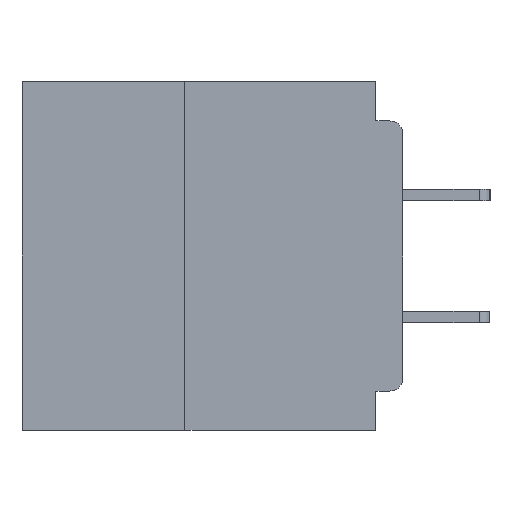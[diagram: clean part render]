
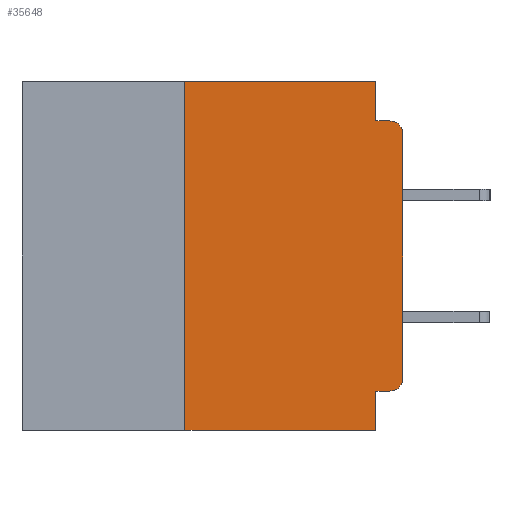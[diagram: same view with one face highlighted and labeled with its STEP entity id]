
A CAD part, left-side view. The second image highlights one B-rep face of the part: STEP entity #35648.
In plain terms, the highlighted planar face has unit normal (-1, 0, 0).
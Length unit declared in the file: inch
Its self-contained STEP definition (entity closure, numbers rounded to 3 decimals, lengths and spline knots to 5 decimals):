
#379 = EDGE_CURVE ( 'NONE', #28760, #12139, #10745, .T. ) ;
#477 = DIRECTION ( 'NONE',  ( 0., 0., 1. ) ) ;
#752 = VECTOR ( 'NONE', #17042, 39.37008 ) ;
#1102 = EDGE_CURVE ( 'NONE', #30086, #15350, #31652, .T. ) ;
#1148 = CARTESIAN_POINT ( 'NONE',  ( 0., 0.25, -0.4 ) ) ;
#1332 = ORIENTED_EDGE ( 'NONE', *, *, #379, .F. ) ;
#1874 = VECTOR ( 'NONE', #34496, 39.37008 ) ;
#2304 = DIRECTION ( 'NONE',  ( 0., 1., 0. ) ) ;
#2606 = LINE ( 'NONE', #16380, #752 ) ;
#2847 = CARTESIAN_POINT ( 'NONE',  ( 0., 0., -0.355 ) ) ;
#2951 = DIRECTION ( 'NONE',  ( 0., -1., 0. ) ) ;
#3468 = DIRECTION ( 'NONE',  ( 1., 0., 0. ) ) ;
#3706 = CARTESIAN_POINT ( 'NONE',  ( 0., 0.031, -0.4 ) ) ;
#4306 = VECTOR ( 'NONE', #2951, 39.37008 ) ;
#4552 = ORIENTED_EDGE ( 'NONE', *, *, #7566, .F. ) ;
#5007 = CARTESIAN_POINT ( 'NONE',  ( 0., 0., -0.34 ) ) ;
#5410 = EDGE_CURVE ( 'NONE', #15923, #11881, #2606, .T. ) ;
#6106 = ORIENTED_EDGE ( 'NONE', *, *, #32459, .T. ) ;
#6788 = EDGE_CURVE ( 'NONE', #8379, #30281, #9928, .T. ) ;
#7203 = EDGE_CURVE ( 'NONE', #11881, #18662, #31814, .T. ) ;
#7566 = EDGE_CURVE ( 'NONE', #12412, #28760, #35286, .T. ) ;
#7842 = EDGE_CURVE ( 'NONE', #30281, #18662, #17129, .T. ) ;
#7962 = EDGE_CURVE ( 'NONE', #12412, #8379, #21242, .T. ) ;
#7987 = CARTESIAN_POINT ( 'NONE',  ( 0., 0.015, -0.045 ) ) ;
#8293 = ORIENTED_EDGE ( 'NONE', *, *, #1102, .F. ) ;
#8379 = VERTEX_POINT ( 'NONE', #5007 ) ;
#8835 = DIRECTION ( 'NONE',  ( 0., 0., -1. ) ) ;
#8938 = CARTESIAN_POINT ( 'NONE',  ( 0., 0.031, -0.045 ) ) ;
#8981 = DIRECTION ( 'NONE',  ( -1., 0., 0. ) ) ;
#9009 = CARTESIAN_POINT ( 'NONE',  ( 0., 0.015, -0.34 ) ) ;
#9731 = VECTOR ( 'NONE', #477, 39.37008 ) ;
#9914 = DIRECTION ( 'NONE',  ( 0., 0., 1. ) ) ;
#9928 = LINE ( 'NONE', #10105, #16770 ) ;
#10105 = CARTESIAN_POINT ( 'NONE',  ( 0., 0., 0. ) ) ;
#10274 = AXIS2_PLACEMENT_3D ( 'NONE', #17454, #17327, #17278 ) ;
#10745 = LINE ( 'NONE', #3706, #1874 ) ;
#10954 = ORIENTED_EDGE ( 'NONE', *, *, #5410, .F. ) ;
#11767 = CARTESIAN_POINT ( 'NONE',  ( 0., 0., -0.06 ) ) ;
#11881 = VERTEX_POINT ( 'NONE', #8938 ) ;
#12139 = VERTEX_POINT ( 'NONE', #36090 ) ;
#12412 = VERTEX_POINT ( 'NONE', #23268 ) ;
#12606 = VECTOR ( 'NONE', #2304, 39.37008 ) ;
#13993 = ORIENTED_EDGE ( 'NONE', *, *, #29779, .F. ) ;
#14252 = ORIENTED_EDGE ( 'NONE', *, *, #6788, .T. ) ;
#15350 = VERTEX_POINT ( 'NONE', #33394 ) ;
#15496 = ORIENTED_EDGE ( 'NONE', *, *, #7203, .F. ) ;
#15923 = VERTEX_POINT ( 'NONE', #21851 ) ;
#15999 = CARTESIAN_POINT ( 'NONE',  ( 0., 0., -0.045 ) ) ;
#16330 = DIRECTION ( 'NONE',  ( 0., -1., 0. ) ) ;
#16375 = DIRECTION ( 'NONE',  ( 0., -1., 0. ) ) ;
#16380 = CARTESIAN_POINT ( 'NONE',  ( 0., 0.031, 0. ) ) ;
#16607 = VECTOR ( 'NONE', #16330, 39.37008 ) ;
#16770 = VECTOR ( 'NONE', #9914, 39.37008 ) ;
#17042 = DIRECTION ( 'NONE',  ( 0., 0., -1. ) ) ;
#17129 = CIRCLE ( 'NONE', #10274, 0.015 ) ;
#17278 = DIRECTION ( 'NONE',  ( 0., 0., -1. ) ) ;
#17327 = DIRECTION ( 'NONE',  ( -1., 0., 0. ) ) ;
#17454 = CARTESIAN_POINT ( 'NONE',  ( 0., 0.015, -0.06 ) ) ;
#17513 = LINE ( 'NONE', #33315, #16607 ) ;
#18129 = LINE ( 'NONE', #37202, #4306 ) ;
#18149 = CARTESIAN_POINT ( 'NONE',  ( 0., 0.437, 0. ) ) ;
#18662 = VERTEX_POINT ( 'NONE', #7987 ) ;
#19388 = CARTESIAN_POINT ( 'NONE',  ( 0., 0.25, -0.4 ) ) ;
#21242 = CIRCLE ( 'NONE', #33248, 0.015 ) ;
#21851 = CARTESIAN_POINT ( 'NONE',  ( 0., 0.031, 0. ) ) ;
#23268 = CARTESIAN_POINT ( 'NONE',  ( 0., 0.015, -0.355 ) ) ;
#23966 = DIRECTION ( 'NONE',  ( 0., 0., -1. ) ) ;
#24332 = EDGE_LOOP ( 'NONE', ( #14252, #34670, #15496, #10954, #13993, #8293, #6106, #1332, #4552, #29966 ) ) ;
#24396 = VECTOR ( 'NONE', #16375, 39.37008 ) ;
#26371 = AXIS2_PLACEMENT_3D ( 'NONE', #18149, #3468, #23966 ) ;
#28760 = VERTEX_POINT ( 'NONE', #33297 ) ;
#28849 = FACE_OUTER_BOUND ( 'NONE', #24332, .T. ) ;
#29779 = EDGE_CURVE ( 'NONE', #15350, #15923, #18129, .T. ) ;
#29966 = ORIENTED_EDGE ( 'NONE', *, *, #7962, .T. ) ;
#30086 = VERTEX_POINT ( 'NONE', #19388 ) ;
#30281 = VERTEX_POINT ( 'NONE', #11767 ) ;
#31652 = LINE ( 'NONE', #1148, #9731 ) ;
#31814 = LINE ( 'NONE', #15999, #24396 ) ;
#32459 = EDGE_CURVE ( 'NONE', #30086, #12139, #17513, .T. ) ;
#33248 = AXIS2_PLACEMENT_3D ( 'NONE', #9009, #8981, #8835 ) ;
#33297 = CARTESIAN_POINT ( 'NONE',  ( 0., 0.031, -0.355 ) ) ;
#33315 = CARTESIAN_POINT ( 'NONE',  ( 0., 0.437, -0.4 ) ) ;
#33394 = CARTESIAN_POINT ( 'NONE',  ( 0., 0.25, 0. ) ) ;
#34496 = DIRECTION ( 'NONE',  ( 0., 0., -1. ) ) ;
#34670 = ORIENTED_EDGE ( 'NONE', *, *, #7842, .T. ) ;
#35044 = PLANE ( 'NONE',  #26371 ) ;
#35286 = LINE ( 'NONE', #2847, #12606 ) ;
#35648 = ADVANCED_FACE ( 'NONE', ( #28849 ), #35044, .F. ) ;
#36090 = CARTESIAN_POINT ( 'NONE',  ( 0., 0.031, -0.4 ) ) ;
#37202 = CARTESIAN_POINT ( 'NONE',  ( 0., 0.437, 0. ) ) ;
